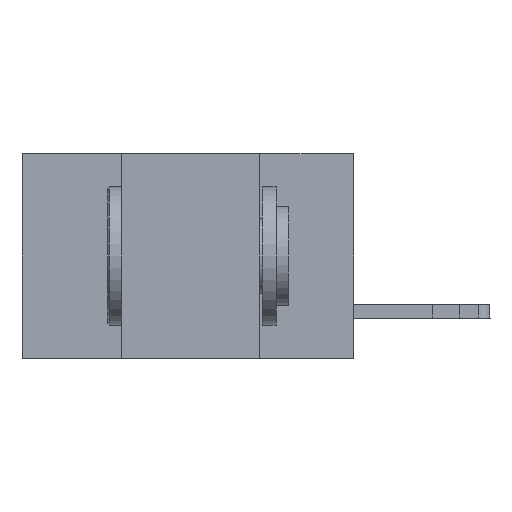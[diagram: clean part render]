
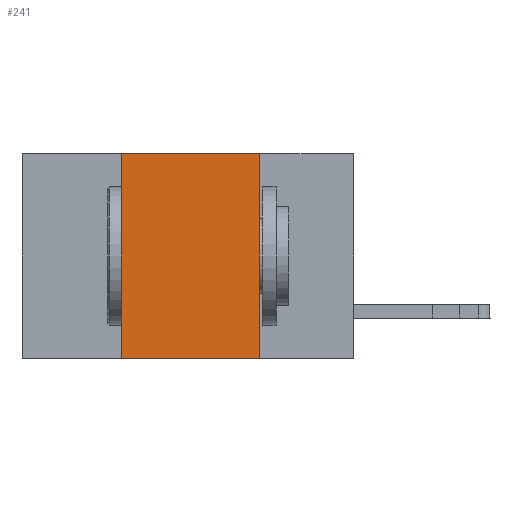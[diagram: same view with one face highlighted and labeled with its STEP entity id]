
A CAD part, left-side view. The second image highlights one B-rep face of the part: STEP entity #241.
In plain terms, the highlighted planar face has unit normal (-1, 0, 0).
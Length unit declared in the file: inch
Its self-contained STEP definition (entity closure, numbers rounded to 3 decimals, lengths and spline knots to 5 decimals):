
#158 = ORIENTED_EDGE ( 'NONE', *, *, #12462, .F. ) ;
#241 = ADVANCED_FACE ( 'NONE', ( #17248 ), #27561, .F. ) ;
#517 = VERTEX_POINT ( 'NONE', #11214 ) ;
#802 = EDGE_CURVE ( 'NONE', #23420, #6866, #12519, .T. ) ;
#1595 = ORIENTED_EDGE ( 'NONE', *, *, #20534, .F. ) ;
#2341 = CARTESIAN_POINT ( 'NONE',  ( 0., 0.42, 0. ) ) ;
#4669 = VECTOR ( 'NONE', #20818, 39.37008 ) ;
#6018 = ORIENTED_EDGE ( 'NONE', *, *, #802, .F. ) ;
#6332 = VERTEX_POINT ( 'NONE', #38302 ) ;
#6866 = VERTEX_POINT ( 'NONE', #35003 ) ;
#11210 = AXIS2_PLACEMENT_3D ( 'NONE', #27768, #29646, #29862 ) ;
#11214 = CARTESIAN_POINT ( 'NONE',  ( 0., 0.42, 0. ) ) ;
#12462 = EDGE_CURVE ( 'NONE', #6332, #517, #36640, .T. ) ;
#12519 = LINE ( 'NONE', #21123, #4669 ) ;
#14028 = LINE ( 'NONE', #26477, #20996 ) ;
#15983 = ORIENTED_EDGE ( 'NONE', *, *, #23684, .T. ) ;
#16169 = VECTOR ( 'NONE', #17001, 39.37008 ) ;
#17001 = DIRECTION ( 'NONE',  ( 0., -1., 0. ) ) ;
#17248 = FACE_OUTER_BOUND ( 'NONE', #30442, .T. ) ;
#20534 = EDGE_CURVE ( 'NONE', #517, #23420, #25027, .T. ) ;
#20818 = DIRECTION ( 'NONE',  ( 0., 0., -1. ) ) ;
#20996 = VECTOR ( 'NONE', #38324, 39.37008 ) ;
#21123 = CARTESIAN_POINT ( 'NONE',  ( 0., 0.17, 0. ) ) ;
#23420 = VERTEX_POINT ( 'NONE', #28266 ) ;
#23684 = EDGE_CURVE ( 'NONE', #6332, #6866, #14028, .T. ) ;
#25027 = LINE ( 'NONE', #25742, #16169 ) ;
#25742 = CARTESIAN_POINT ( 'NONE',  ( 0., 0.6, 0. ) ) ;
#26477 = CARTESIAN_POINT ( 'NONE',  ( 0., 0.6, -0.37 ) ) ;
#27561 = PLANE ( 'NONE',  #11210 ) ;
#27768 = CARTESIAN_POINT ( 'NONE',  ( 0., 0.6, 0. ) ) ;
#28266 = CARTESIAN_POINT ( 'NONE',  ( 0., 0.17, 0. ) ) ;
#29646 = DIRECTION ( 'NONE',  ( 1., 0., 0. ) ) ;
#29680 = VECTOR ( 'NONE', #31994, 39.37008 ) ;
#29862 = DIRECTION ( 'NONE',  ( 0., 0., -1. ) ) ;
#30442 = EDGE_LOOP ( 'NONE', ( #6018, #1595, #158, #15983 ) ) ;
#31994 = DIRECTION ( 'NONE',  ( 0., 0., 1. ) ) ;
#35003 = CARTESIAN_POINT ( 'NONE',  ( 0., 0.17, -0.37 ) ) ;
#36640 = LINE ( 'NONE', #2341, #29680 ) ;
#38302 = CARTESIAN_POINT ( 'NONE',  ( 0., 0.42, -0.37 ) ) ;
#38324 = DIRECTION ( 'NONE',  ( 0., -1., 0. ) ) ;
